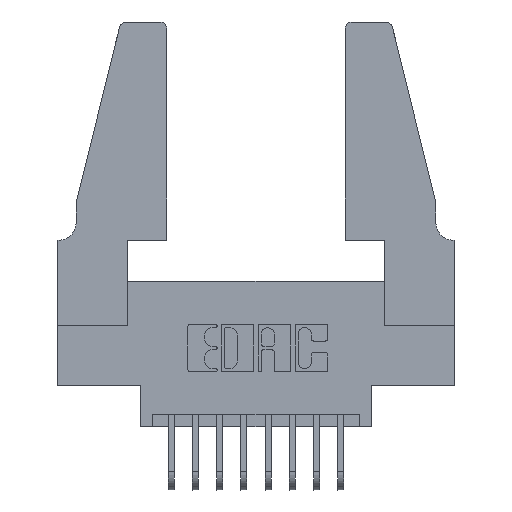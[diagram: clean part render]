
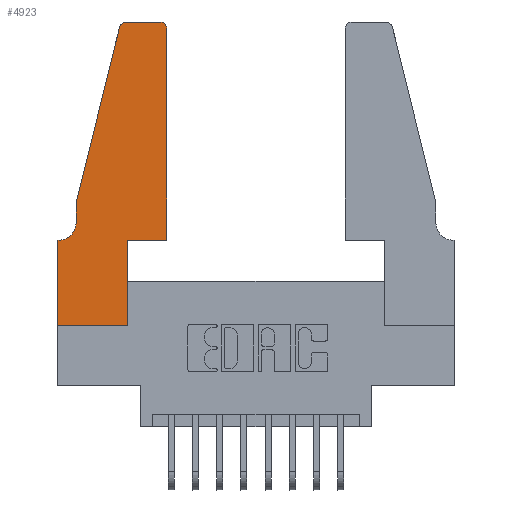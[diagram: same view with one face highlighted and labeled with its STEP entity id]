
A CAD part, top view. The second image highlights one B-rep face of the part: STEP entity #4923.
In plain terms, the highlighted planar face has unit normal (0, 0, 1).
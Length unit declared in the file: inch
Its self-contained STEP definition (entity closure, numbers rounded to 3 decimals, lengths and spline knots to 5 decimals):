
#76 = DIRECTION ( 'NONE',  ( -1., 0., 0. ) ) ;
#210 = CARTESIAN_POINT ( 'NONE',  ( 0.284, 1.22, 0.37 ) ) ;
#313 = DIRECTION ( 'NONE',  ( 0., -1., 0. ) ) ;
#522 = CARTESIAN_POINT ( 'NONE',  ( 0.4505, 0.35, 0.37 ) ) ;
#742 = CARTESIAN_POINT ( 'NONE',  ( 0.0755, 0.5, 0.37 ) ) ;
#924 = VERTEX_POINT ( 'NONE', #3341 ) ;
#1034 = VERTEX_POINT ( 'NONE', #3750 ) ;
#1382 = DIRECTION ( 'NONE',  ( 1., 0., 0. ) ) ;
#1426 = CARTESIAN_POINT ( 'NONE',  ( 0., 0., 0.37 ) ) ;
#1498 = ORIENTED_EDGE ( 'NONE', *, *, #8456, .T. ) ;
#1550 = CARTESIAN_POINT ( 'NONE',  ( 0.0055, 0.42, 0.37 ) ) ;
#1640 = DIRECTION ( 'NONE',  ( 0., -1., 0. ) ) ;
#1667 = EDGE_CURVE ( 'NONE', #1867, #4702, #12118, .T. ) ;
#1867 = VERTEX_POINT ( 'NONE', #13960 ) ;
#1949 = ORIENTED_EDGE ( 'NONE', *, *, #13624, .T. ) ;
#1997 = ORIENTED_EDGE ( 'NONE', *, *, #1667, .T. ) ;
#2041 = CARTESIAN_POINT ( 'NONE',  ( 0.0755, 0.35, 0.37 ) ) ;
#2231 = AXIS2_PLACEMENT_3D ( 'NONE', #210, #8394, #1382 ) ;
#2348 = VERTEX_POINT ( 'NONE', #10595 ) ;
#2351 = ORIENTED_EDGE ( 'NONE', *, *, #4463, .T. ) ;
#2434 = CARTESIAN_POINT ( 'NONE',  ( 0.2605, 1.25, 0.37 ) ) ;
#2627 = CARTESIAN_POINT ( 'NONE',  ( 0., 0., 0.37 ) ) ;
#2639 = DIRECTION ( 'NONE',  ( -1., 0., 0. ) ) ;
#2673 = LINE ( 'NONE', #2041, #5397 ) ;
#2740 = DIRECTION ( 'NONE',  ( -1., 0., 0. ) ) ;
#2942 = ORIENTED_EDGE ( 'NONE', *, *, #6614, .T. ) ;
#3030 = EDGE_CURVE ( 'NONE', #9002, #1867, #9811, .T. ) ;
#3200 = CARTESIAN_POINT ( 'NONE',  ( 0.4505, 0.35, 0.37 ) ) ;
#3217 = VECTOR ( 'NONE', #11230, 39.37008 ) ;
#3341 = CARTESIAN_POINT ( 'NONE',  ( 0.0755, 0.42, 0.37 ) ) ;
#3507 = CARTESIAN_POINT ( 'NONE',  ( 0.0055, 0.35, 0.37 ) ) ;
#3750 = CARTESIAN_POINT ( 'NONE',  ( 0.4505, 0.35, 0.37 ) ) ;
#3835 = DIRECTION ( 'NONE',  ( 0., 0., 1. ) ) ;
#3860 = EDGE_CURVE ( 'NONE', #8846, #9520, #2673, .T. ) ;
#3936 = FACE_OUTER_BOUND ( 'NONE', #7611, .T. ) ;
#3970 = CARTESIAN_POINT ( 'NONE',  ( 0.0755, 0.5, 0.37 ) ) ;
#4197 = CARTESIAN_POINT ( 'NONE',  ( 0.4505, 1.22, 0.37 ) ) ;
#4463 = EDGE_CURVE ( 'NONE', #2348, #11907, #6292, .T. ) ;
#4466 = VECTOR ( 'NONE', #7540, 39.37008 ) ;
#4479 = VECTOR ( 'NONE', #1640, 39.37008 ) ;
#4702 = VERTEX_POINT ( 'NONE', #11642 ) ;
#4713 = CARTESIAN_POINT ( 'NONE',  ( 0., 0.35, 0.37 ) ) ;
#4814 = LINE ( 'NONE', #522, #4466 ) ;
#4860 = LINE ( 'NONE', #3200, #12910 ) ;
#4923 = ADVANCED_FACE ( 'NONE', ( #3936 ), #6462, .T. ) ;
#5282 = CARTESIAN_POINT ( 'NONE',  ( 0.4205, 1.25, 0.37 ) ) ;
#5397 = VECTOR ( 'NONE', #2639, 39.37008 ) ;
#5490 = EDGE_CURVE ( 'NONE', #4702, #1034, #4814, .T. ) ;
#5519 = DIRECTION ( 'NONE',  ( 0., 1., 0. ) ) ;
#5671 = VECTOR ( 'NONE', #76, 39.37008 ) ;
#5776 = LINE ( 'NONE', #2627, #11558 ) ;
#6292 = LINE ( 'NONE', #742, #3217 ) ;
#6462 = PLANE ( 'NONE',  #8589 ) ;
#6614 = EDGE_CURVE ( 'NONE', #8581, #11032, #14698, .T. ) ;
#7083 = VECTOR ( 'NONE', #11610, 39.37008 ) ;
#7540 = DIRECTION ( 'NONE',  ( 1., 0., 0. ) ) ;
#7586 = LINE ( 'NONE', #3970, #4479 ) ;
#7611 = EDGE_LOOP ( 'NONE', ( #2942, #9823, #2351, #12785, #1498, #13662, #8552, #7714, #1997, #10391, #1949, #9479 ) ) ;
#7660 = DIRECTION ( 'NONE',  ( 1., 0., 0. ) ) ;
#7714 = ORIENTED_EDGE ( 'NONE', *, *, #3030, .T. ) ;
#8394 = DIRECTION ( 'NONE',  ( 0., 0., 1. ) ) ;
#8456 = EDGE_CURVE ( 'NONE', #924, #8846, #9450, .T. ) ;
#8552 = ORIENTED_EDGE ( 'NONE', *, *, #13292, .T. ) ;
#8581 = VERTEX_POINT ( 'NONE', #5282 ) ;
#8589 = AXIS2_PLACEMENT_3D ( 'NONE', #13275, #14342, #7660 ) ;
#8731 = AXIS2_PLACEMENT_3D ( 'NONE', #1550, #9725, #2740 ) ;
#8773 = VECTOR ( 'NONE', #14809, 39.37008 ) ;
#8846 = VERTEX_POINT ( 'NONE', #3507 ) ;
#8897 = CIRCLE ( 'NONE', #2231, 0.03 ) ;
#9002 = VERTEX_POINT ( 'NONE', #1426 ) ;
#9450 = CIRCLE ( 'NONE', #8731, 0.07 ) ;
#9479 = ORIENTED_EDGE ( 'NONE', *, *, #10752, .T. ) ;
#9517 = AXIS2_PLACEMENT_3D ( 'NONE', #10768, #3835, #11877 ) ;
#9520 = VERTEX_POINT ( 'NONE', #4713 ) ;
#9547 = CARTESIAN_POINT ( 'NONE',  ( 0.0755, 0.5, 0.37 ) ) ;
#9725 = DIRECTION ( 'NONE',  ( 0., 0., -1. ) ) ;
#9811 = LINE ( 'NONE', #11771, #7083 ) ;
#9823 = ORIENTED_EDGE ( 'NONE', *, *, #13253, .T. ) ;
#9853 = VERTEX_POINT ( 'NONE', #4197 ) ;
#10391 = ORIENTED_EDGE ( 'NONE', *, *, #5490, .T. ) ;
#10595 = CARTESIAN_POINT ( 'NONE',  ( 0.25487, 1.22718, 0.37 ) ) ;
#10752 = EDGE_CURVE ( 'NONE', #9853, #8581, #13259, .T. ) ;
#10768 = CARTESIAN_POINT ( 'NONE',  ( 0.4205, 1.22, 0.37 ) ) ;
#11032 = VERTEX_POINT ( 'NONE', #13476 ) ;
#11230 = DIRECTION ( 'NONE',  ( -0.239, -0.971, 0. ) ) ;
#11509 = EDGE_CURVE ( 'NONE', #11907, #924, #7586, .T. ) ;
#11558 = VECTOR ( 'NONE', #313, 39.37008 ) ;
#11610 = DIRECTION ( 'NONE',  ( 1., 0., 0. ) ) ;
#11642 = CARTESIAN_POINT ( 'NONE',  ( 0.2865, 0.35, 0.37 ) ) ;
#11771 = CARTESIAN_POINT ( 'NONE',  ( 0., 0., 0.37 ) ) ;
#11877 = DIRECTION ( 'NONE',  ( 1., 0., 0. ) ) ;
#11907 = VERTEX_POINT ( 'NONE', #9547 ) ;
#12118 = LINE ( 'NONE', #12641, #8773 ) ;
#12641 = CARTESIAN_POINT ( 'NONE',  ( 0.2865, 0.35, 0.37 ) ) ;
#12785 = ORIENTED_EDGE ( 'NONE', *, *, #11509, .T. ) ;
#12910 = VECTOR ( 'NONE', #5519, 39.37008 ) ;
#13253 = EDGE_CURVE ( 'NONE', #11032, #2348, #8897, .T. ) ;
#13259 = CIRCLE ( 'NONE', #9517, 0.03 ) ;
#13275 = CARTESIAN_POINT ( 'NONE',  ( 0., 0.35, 0.37 ) ) ;
#13292 = EDGE_CURVE ( 'NONE', #9520, #9002, #5776, .T. ) ;
#13476 = CARTESIAN_POINT ( 'NONE',  ( 0.284, 1.25, 0.37 ) ) ;
#13624 = EDGE_CURVE ( 'NONE', #1034, #9853, #4860, .T. ) ;
#13662 = ORIENTED_EDGE ( 'NONE', *, *, #3860, .T. ) ;
#13960 = CARTESIAN_POINT ( 'NONE',  ( 0.2865, 0., 0.37 ) ) ;
#14342 = DIRECTION ( 'NONE',  ( 0., 0., 1. ) ) ;
#14698 = LINE ( 'NONE', #2434, #5671 ) ;
#14809 = DIRECTION ( 'NONE',  ( 0., 1., 0. ) ) ;
